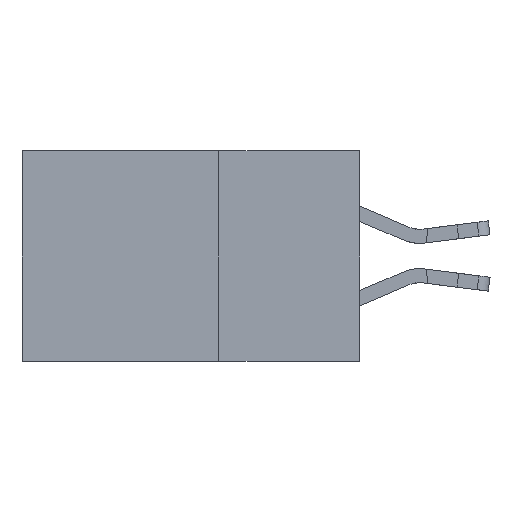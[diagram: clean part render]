
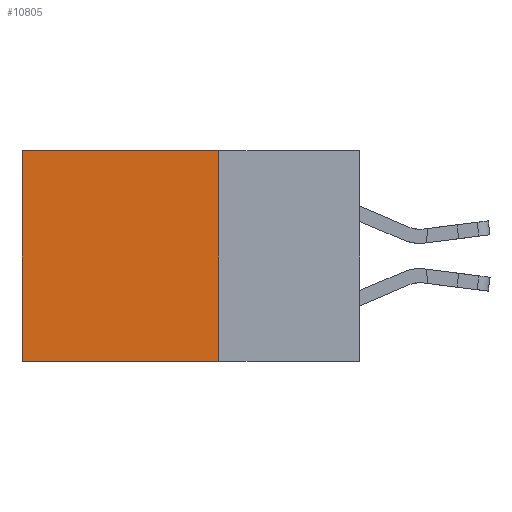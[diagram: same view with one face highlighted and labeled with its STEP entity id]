
A CAD part, left-side view. The second image highlights one B-rep face of the part: STEP entity #10805.
In plain terms, the highlighted planar face has unit normal (-1, 0, 0).
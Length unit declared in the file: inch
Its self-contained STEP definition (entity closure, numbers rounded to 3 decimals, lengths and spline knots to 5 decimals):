
#509 = DIRECTION ( 'NONE',  ( 0., 1., 0. ) ) ;
#1678 = CARTESIAN_POINT ( 'NONE',  ( 0.2875, 0.6, -0.375 ) ) ;
#2189 = DIRECTION ( 'NONE',  ( 0., 0., -1. ) ) ;
#2579 = EDGE_CURVE ( 'NONE', #9212, #4110, #13772, .T. ) ;
#2830 = DIRECTION ( 'NONE',  ( 0., 0., -1. ) ) ;
#3527 = DIRECTION ( 'NONE',  ( 0., 0., -1. ) ) ;
#4110 = VERTEX_POINT ( 'NONE', #1678 ) ;
#4325 = LINE ( 'NONE', #16221, #7527 ) ;
#5550 = FACE_OUTER_BOUND ( 'NONE', #8715, .T. ) ;
#5913 = ORIENTED_EDGE ( 'NONE', *, *, #9790, .T. ) ;
#6393 = EDGE_CURVE ( 'NONE', #16866, #4110, #12427, .T. ) ;
#6584 = VERTEX_POINT ( 'NONE', #8195 ) ;
#7527 = VECTOR ( 'NONE', #509, 39.37008 ) ;
#7785 = VECTOR ( 'NONE', #2189, 39.37008 ) ;
#8119 = ORIENTED_EDGE ( 'NONE', *, *, #18542, .F. ) ;
#8195 = CARTESIAN_POINT ( 'NONE',  ( 0.2875, 0.25, 0. ) ) ;
#8715 = EDGE_LOOP ( 'NONE', ( #15025, #15042, #8119, #5913 ) ) ;
#8780 = DIRECTION ( 'NONE',  ( 0., 1., 0. ) ) ;
#9212 = VERTEX_POINT ( 'NONE', #13770 ) ;
#9647 = VECTOR ( 'NONE', #8780, 39.37008 ) ;
#9656 = DIRECTION ( 'NONE',  ( 1., 0., 0. ) ) ;
#9790 = EDGE_CURVE ( 'NONE', #6584, #16866, #4325, .T. ) ;
#10381 = CARTESIAN_POINT ( 'NONE',  ( 0.2875, 0.6, 0. ) ) ;
#10805 = ADVANCED_FACE ( 'NONE', ( #5550 ), #14202, .F. ) ;
#10819 = CARTESIAN_POINT ( 'NONE',  ( 0.2875, 0.25, -0.375 ) ) ;
#11608 = CARTESIAN_POINT ( 'NONE',  ( 0.2875, 0.6, -0.375 ) ) ;
#11885 = VECTOR ( 'NONE', #2830, 39.37008 ) ;
#12427 = LINE ( 'NONE', #11608, #7785 ) ;
#12982 = CARTESIAN_POINT ( 'NONE',  ( 0.2875, 0.25, -0.375 ) ) ;
#13770 = CARTESIAN_POINT ( 'NONE',  ( 0.2875, 0.25, -0.375 ) ) ;
#13772 = LINE ( 'NONE', #15053, #9647 ) ;
#14202 = PLANE ( 'NONE',  #14922 ) ;
#14568 = LINE ( 'NONE', #10819, #11885 ) ;
#14922 = AXIS2_PLACEMENT_3D ( 'NONE', #12982, #9656, #3527 ) ;
#15025 = ORIENTED_EDGE ( 'NONE', *, *, #6393, .T. ) ;
#15042 = ORIENTED_EDGE ( 'NONE', *, *, #2579, .F. ) ;
#15053 = CARTESIAN_POINT ( 'NONE',  ( 0.2875, 0.25, -0.375 ) ) ;
#16221 = CARTESIAN_POINT ( 'NONE',  ( 0.2875, 0.25, 0. ) ) ;
#16866 = VERTEX_POINT ( 'NONE', #10381 ) ;
#18542 = EDGE_CURVE ( 'NONE', #6584, #9212, #14568, .T. ) ;
